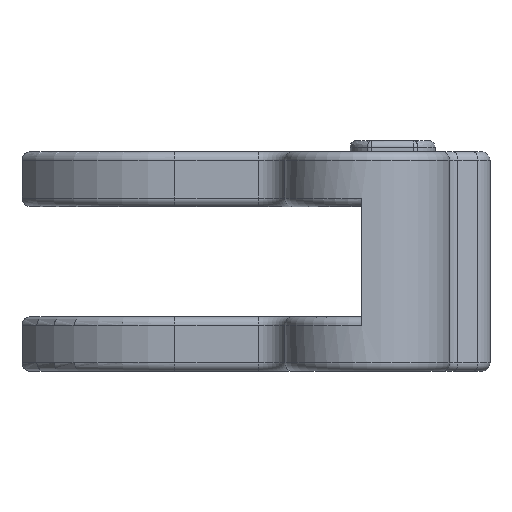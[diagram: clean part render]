
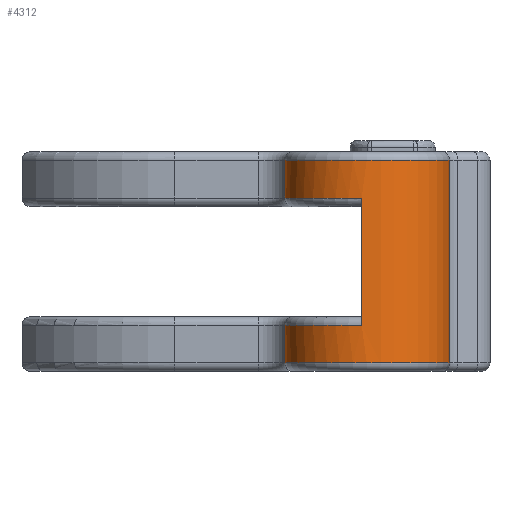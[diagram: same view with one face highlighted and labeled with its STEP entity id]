
A CAD part, front view. The second image highlights one B-rep face of the part: STEP entity #4312.
In plain terms, the highlighted cylindrical face has radius 9.538 mm (diameter 19.075 mm), a partial arc.
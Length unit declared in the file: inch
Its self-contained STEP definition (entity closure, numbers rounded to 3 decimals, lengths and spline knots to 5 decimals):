
#27 = VERTEX_POINT ( 'NONE', #4834 ) ;
#249 = DIRECTION ( 'NONE',  ( 0., 0., -1. ) ) ;
#267 = CARTESIAN_POINT ( 'NONE',  ( 0.24661, -0.96897, 0.08013 ) ) ;
#454 = CARTESIAN_POINT ( 'NONE',  ( -0.1259, -0.9217, -0.09113 ) ) ;
#593 = ORIENTED_EDGE ( 'NONE', *, *, #4331, .T. ) ;
#633 = EDGE_CURVE ( 'NONE', #27, #862, #4849, .T. ) ;
#722 = ORIENTED_EDGE ( 'NONE', *, *, #944, .T. ) ;
#733 = DIRECTION ( 'NONE',  ( 1., 0., 0. ) ) ;
#743 = DIRECTION ( 'NONE',  ( 0., 0., 1. ) ) ;
#744 = CARTESIAN_POINT ( 'NONE',  ( 0.24661, -0.96897, -0.09113 ) ) ;
#755 = EDGE_CURVE ( 'NONE', #4495, #27, #4733, .T. ) ;
#803 = DIRECTION ( 'NONE',  ( 0., 0., -1. ) ) ;
#847 = CARTESIAN_POINT ( 'NONE',  ( 0.24661, -0.96897, -0.66987 ) ) ;
#862 = VERTEX_POINT ( 'NONE', #1397 ) ;
#900 = CARTESIAN_POINT ( 'NONE',  ( 0.221, -1.34359, 3.60324 ) ) ;
#944 = EDGE_CURVE ( 'NONE', #1380, #4730, #4671, .T. ) ;
#1062 = ORIENTED_EDGE ( 'NONE', *, *, #1090, .T. ) ;
#1090 = EDGE_CURVE ( 'NONE', #862, #3304, #4577, .T. ) ;
#1121 = CARTESIAN_POINT ( 'NONE',  ( 0.24661, -0.96897, 3.60324 ) ) ;
#1164 = DIRECTION ( 'NONE',  ( -1., 0., 0. ) ) ;
#1380 = VERTEX_POINT ( 'NONE', #1652 ) ;
#1397 = CARTESIAN_POINT ( 'NONE',  ( 0.60744, -0.86504, -0.84113 ) ) ;
#1413 = DIRECTION ( 'NONE',  ( -1., 0., 0. ) ) ;
#1618 = AXIS2_PLACEMENT_3D ( 'NONE', #267, #249, #2082 ) ;
#1652 = CARTESIAN_POINT ( 'NONE',  ( -0.1259, -0.9217, 0.08013 ) ) ;
#1693 = AXIS2_PLACEMENT_3D ( 'NONE', #4028, #4023, #4021 ) ;
#1709 = EDGE_CURVE ( 'NONE', #4730, #2780, #4330, .T. ) ;
#1753 = ORIENTED_EDGE ( 'NONE', *, *, #1709, .T. ) ;
#1995 = ORIENTED_EDGE ( 'NONE', *, *, #2968, .T. ) ;
#2082 = DIRECTION ( 'NONE',  ( 1., 0., 0. ) ) ;
#2111 = ORIENTED_EDGE ( 'NONE', *, *, #633, .T. ) ;
#2117 = CARTESIAN_POINT ( 'NONE',  ( 0.60744, -0.86504, 3.60324 ) ) ;
#2145 = EDGE_CURVE ( 'NONE', #2780, #2868, #4091, .T. ) ;
#2371 = DIRECTION ( 'NONE',  ( 0., 0., 1. ) ) ;
#2543 = CIRCLE ( 'NONE', #1618, 0.3755 ) ;
#2562 = CYLINDRICAL_SURFACE ( 'NONE', #3703, 0.3755 ) ;
#2600 = FACE_OUTER_BOUND ( 'NONE', #4412, .T. ) ;
#2707 = DIRECTION ( 'NONE',  ( 0., 0., -1. ) ) ;
#2780 = VERTEX_POINT ( 'NONE', #2824 ) ;
#2824 = CARTESIAN_POINT ( 'NONE',  ( 0.221, -1.34359, -0.09113 ) ) ;
#2868 = VERTEX_POINT ( 'NONE', #3701 ) ;
#2968 = EDGE_CURVE ( 'NONE', #2868, #4495, #3773, .T. ) ;
#2998 = DIRECTION ( 'NONE',  ( 0., 0., -1. ) ) ;
#3115 = CARTESIAN_POINT ( 'NONE',  ( 0.60744, -0.86504, 0.08013 ) ) ;
#3138 = CARTESIAN_POINT ( 'NONE',  ( -0.1259, -0.9217, 3.60324 ) ) ;
#3304 = VERTEX_POINT ( 'NONE', #3115 ) ;
#3371 = DIRECTION ( 'NONE',  ( 0., 0., -1. ) ) ;
#3391 = CARTESIAN_POINT ( 'NONE',  ( -0.1259, -0.9217, 3.60324 ) ) ;
#3460 = DIRECTION ( 'NONE',  ( 0., 0., -1. ) ) ;
#3585 = AXIS2_PLACEMENT_3D ( 'NONE', #847, #3371, #1164 ) ;
#3592 = ORIENTED_EDGE ( 'NONE', *, *, #2145, .T. ) ;
#3701 = CARTESIAN_POINT ( 'NONE',  ( 0.221, -1.34359, -0.66987 ) ) ;
#3703 = AXIS2_PLACEMENT_3D ( 'NONE', #1121, #803, #1413 ) ;
#3773 = CIRCLE ( 'NONE', #3585, 0.3755 ) ;
#3848 = AXIS2_PLACEMENT_3D ( 'NONE', #744, #743, #733 ) ;
#4021 = DIRECTION ( 'NONE',  ( -1., 0., 0. ) ) ;
#4023 = DIRECTION ( 'NONE',  ( 0., 0., 1. ) ) ;
#4028 = CARTESIAN_POINT ( 'NONE',  ( 0.24661, -0.96897, -0.84113 ) ) ;
#4077 = VECTOR ( 'NONE', #2998, 39.37008 ) ;
#4091 = LINE ( 'NONE', #900, #4077 ) ;
#4312 = ADVANCED_FACE ( 'NONE', ( #2600 ), #2562, .T. ) ;
#4330 = CIRCLE ( 'NONE', #3848, 0.3755 ) ;
#4331 = EDGE_CURVE ( 'NONE', #3304, #1380, #2543, .T. ) ;
#4385 = CARTESIAN_POINT ( 'NONE',  ( -0.1259, -0.9217, -0.66987 ) ) ;
#4388 = ORIENTED_EDGE ( 'NONE', *, *, #755, .T. ) ;
#4412 = EDGE_LOOP ( 'NONE', ( #722, #1753, #3592, #1995, #4388, #2111, #1062, #593 ) ) ;
#4495 = VERTEX_POINT ( 'NONE', #4385 ) ;
#4572 = VECTOR ( 'NONE', #2371, 39.37008 ) ;
#4577 = LINE ( 'NONE', #2117, #4572 ) ;
#4661 = VECTOR ( 'NONE', #2707, 39.37008 ) ;
#4671 = LINE ( 'NONE', #3138, #4661 ) ;
#4730 = VERTEX_POINT ( 'NONE', #454 ) ;
#4732 = VECTOR ( 'NONE', #3460, 39.37008 ) ;
#4733 = LINE ( 'NONE', #3391, #4732 ) ;
#4834 = CARTESIAN_POINT ( 'NONE',  ( -0.1259, -0.9217, -0.84113 ) ) ;
#4849 = CIRCLE ( 'NONE', #1693, 0.3755 ) ;
